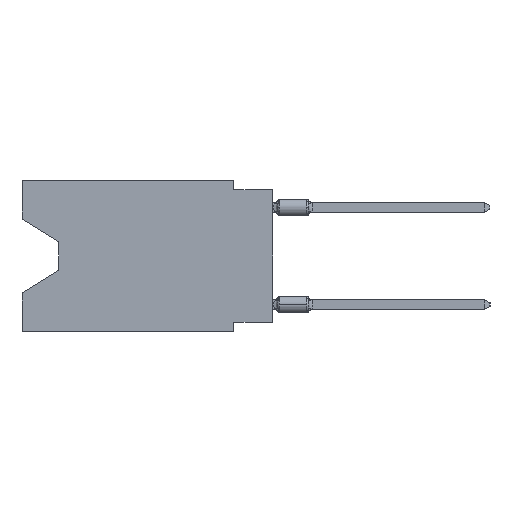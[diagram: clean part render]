
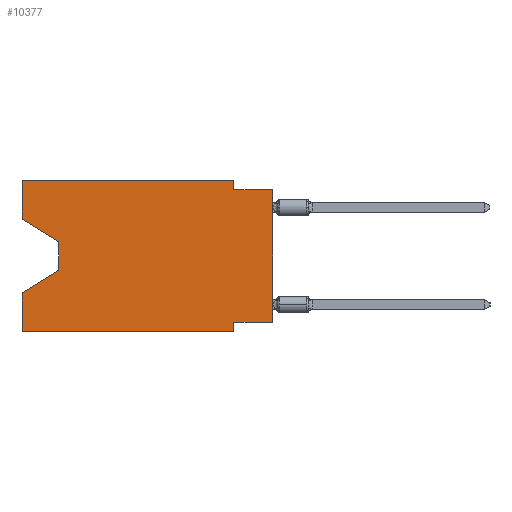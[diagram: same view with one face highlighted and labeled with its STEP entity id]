
A CAD part, left-side view. The second image highlights one B-rep face of the part: STEP entity #10377.
In plain terms, the highlighted planar face has unit normal (-1, 0, 0).
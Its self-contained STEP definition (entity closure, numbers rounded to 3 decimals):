
#88 = LINE ( 'NONE', #32011, #31797 ) ;
#122 = DIRECTION ( 'NONE',  ( 0., 0., 1. ) ) ;
#238 = LINE ( 'NONE', #20340, #31141 ) ;
#294 = DIRECTION ( 'NONE',  ( 0., 1., 0. ) ) ;
#889 = DIRECTION ( 'NONE',  ( 0., 0., -1. ) ) ;
#979 = DIRECTION ( 'NONE',  ( 0., 0.855, -0.519 ) ) ;
#1018 = VECTOR ( 'NONE', #294, 1000. ) ;
#1176 = CARTESIAN_POINT ( 'NONE',  ( 0., 16.383, 0. ) ) ;
#1333 = CARTESIAN_POINT ( 'NONE',  ( 0., 13.97, -4.013 ) ) ;
#1565 = EDGE_CURVE ( 'NONE', #36965, #25003, #2427, .T. ) ;
#2427 = LINE ( 'NONE', #22692, #28258 ) ;
#3397 = CARTESIAN_POINT ( 'NONE',  ( 0., 0., -9.271 ) ) ;
#3689 = CARTESIAN_POINT ( 'NONE',  ( 0., 2.54, -0.635 ) ) ;
#3773 = EDGE_CURVE ( 'NONE', #7853, #16053, #88, .T. ) ;
#4443 = DIRECTION ( 'NONE',  ( 0., 0., 1. ) ) ;
#4765 = VECTOR ( 'NONE', #889, 1000. ) ;
#4847 = VERTEX_POINT ( 'NONE', #28149 ) ;
#4906 = DIRECTION ( 'NONE',  ( 0., 0., -1. ) ) ;
#5166 = VECTOR ( 'NONE', #4443, 1000. ) ;
#5516 = ORIENTED_EDGE ( 'NONE', *, *, #20604, .T. ) ;
#5709 = LINE ( 'NONE', #32572, #13182 ) ;
#6017 = ORIENTED_EDGE ( 'NONE', *, *, #27268, .F. ) ;
#6082 = ORIENTED_EDGE ( 'NONE', *, *, #20113, .T. ) ;
#6728 = LINE ( 'NONE', #30863, #16703 ) ;
#7467 = LINE ( 'NONE', #34521, #18768 ) ;
#7670 = ORIENTED_EDGE ( 'NONE', *, *, #17733, .F. ) ;
#7853 = VERTEX_POINT ( 'NONE', #1333 ) ;
#8431 = DIRECTION ( 'NONE',  ( 0., 0., -1. ) ) ;
#9542 = CARTESIAN_POINT ( 'NONE',  ( 0., 0., -9.271 ) ) ;
#9868 = ORIENTED_EDGE ( 'NONE', *, *, #16961, .F. ) ;
#10208 = ORIENTED_EDGE ( 'NONE', *, *, #37325, .F. ) ;
#10320 = PLANE ( 'NONE',  #21846 ) ;
#10377 = ADVANCED_FACE ( 'NONE', ( #13979 ), #10320, .F. ) ;
#10885 = DIRECTION ( 'NONE',  ( 1., 0., 0. ) ) ;
#11122 = CARTESIAN_POINT ( 'NONE',  ( 0., 2.54, -9.271 ) ) ;
#11382 = ORIENTED_EDGE ( 'NONE', *, *, #1565, .F. ) ;
#12077 = DIRECTION ( 'NONE',  ( 0., -1., 0. ) ) ;
#12744 = LINE ( 'NONE', #33243, #15649 ) ;
#12853 = LINE ( 'NONE', #21547, #4765 ) ;
#12995 = VERTEX_POINT ( 'NONE', #36056 ) ;
#13182 = VECTOR ( 'NONE', #35274, 1000. ) ;
#13979 = FACE_OUTER_BOUND ( 'NONE', #22973, .T. ) ;
#15639 = ORIENTED_EDGE ( 'NONE', *, *, #19374, .T. ) ;
#15649 = VECTOR ( 'NONE', #979, 1000. ) ;
#16053 = VERTEX_POINT ( 'NONE', #17412 ) ;
#16703 = VECTOR ( 'NONE', #28278, 1000. ) ;
#16961 = EDGE_CURVE ( 'NONE', #12995, #26258, #25131, .T. ) ;
#17412 = CARTESIAN_POINT ( 'NONE',  ( 0., 13.97, -5.893 ) ) ;
#17643 = DIRECTION ( 'NONE',  ( 0., -0.855, -0.519 ) ) ;
#17688 = LINE ( 'NONE', #28387, #28089 ) ;
#17733 = EDGE_CURVE ( 'NONE', #34041, #21862, #26771, .T. ) ;
#18297 = LINE ( 'NONE', #29891, #20986 ) ;
#18768 = VECTOR ( 'NONE', #25828, 1000. ) ;
#19374 = EDGE_CURVE ( 'NONE', #16053, #26258, #12744, .T. ) ;
#19878 = EDGE_CURVE ( 'NONE', #25003, #28937, #7467, .T. ) ;
#20113 = EDGE_CURVE ( 'NONE', #34041, #28937, #5709, .T. ) ;
#20340 = CARTESIAN_POINT ( 'NONE',  ( 0., 16.383, -2.546 ) ) ;
#20567 = CARTESIAN_POINT ( 'NONE',  ( 0., 16.383, -2.546 ) ) ;
#20604 = EDGE_CURVE ( 'NONE', #24262, #7853, #238, .T. ) ;
#20986 = VECTOR ( 'NONE', #122, 1000. ) ;
#21547 = CARTESIAN_POINT ( 'NONE',  ( 0., 2.54, -9.906 ) ) ;
#21846 = AXIS2_PLACEMENT_3D ( 'NONE', #34278, #10885, #4906 ) ;
#21862 = VERTEX_POINT ( 'NONE', #11122 ) ;
#22692 = CARTESIAN_POINT ( 'NONE',  ( 0., 2.54, 0. ) ) ;
#22973 = EDGE_LOOP ( 'NONE', ( #5516, #37723, #15639, #9868, #28539, #6017, #7670, #6082, #28277, #11382, #23898, #10208 ) ) ;
#23240 = CARTESIAN_POINT ( 'NONE',  ( 0., 2.54, -9.906 ) ) ;
#23898 = ORIENTED_EDGE ( 'NONE', *, *, #25287, .F. ) ;
#24262 = VERTEX_POINT ( 'NONE', #20567 ) ;
#25003 = VERTEX_POINT ( 'NONE', #3689 ) ;
#25105 = CARTESIAN_POINT ( 'NONE',  ( 0., 2.54, 0. ) ) ;
#25131 = LINE ( 'NONE', #1176, #5166 ) ;
#25287 = EDGE_CURVE ( 'NONE', #4847, #36965, #17688, .T. ) ;
#25499 = CARTESIAN_POINT ( 'NONE',  ( 0., 16.383, -7.36 ) ) ;
#25828 = DIRECTION ( 'NONE',  ( 0., -1., 0. ) ) ;
#26258 = VERTEX_POINT ( 'NONE', #25499 ) ;
#26771 = LINE ( 'NONE', #3397, #1018 ) ;
#27164 = CARTESIAN_POINT ( 'NONE',  ( 0., 0., -0.635 ) ) ;
#27268 = EDGE_CURVE ( 'NONE', #21862, #36280, #12853, .T. ) ;
#28089 = VECTOR ( 'NONE', #12077, 1000. ) ;
#28149 = CARTESIAN_POINT ( 'NONE',  ( 0., 16.383, 0. ) ) ;
#28258 = VECTOR ( 'NONE', #28886, 1000. ) ;
#28277 = ORIENTED_EDGE ( 'NONE', *, *, #19878, .F. ) ;
#28278 = DIRECTION ( 'NONE',  ( 0., -1., 0. ) ) ;
#28387 = CARTESIAN_POINT ( 'NONE',  ( 0., 16.383, 0. ) ) ;
#28539 = ORIENTED_EDGE ( 'NONE', *, *, #36065, .T. ) ;
#28886 = DIRECTION ( 'NONE',  ( 0., 0., -1. ) ) ;
#28937 = VERTEX_POINT ( 'NONE', #27164 ) ;
#29891 = CARTESIAN_POINT ( 'NONE',  ( 0., 16.383, 0. ) ) ;
#30863 = CARTESIAN_POINT ( 'NONE',  ( 0., 16.383, -9.906 ) ) ;
#31141 = VECTOR ( 'NONE', #17643, 1000. ) ;
#31797 = VECTOR ( 'NONE', #8431, 1000. ) ;
#32011 = CARTESIAN_POINT ( 'NONE',  ( 0., 13.97, -4.013 ) ) ;
#32572 = CARTESIAN_POINT ( 'NONE',  ( 0., 0., 0. ) ) ;
#33243 = CARTESIAN_POINT ( 'NONE',  ( 0., 13.97, -5.893 ) ) ;
#34041 = VERTEX_POINT ( 'NONE', #9542 ) ;
#34278 = CARTESIAN_POINT ( 'NONE',  ( 0., 16.383, 0. ) ) ;
#34521 = CARTESIAN_POINT ( 'NONE',  ( 0., 0., -0.635 ) ) ;
#35274 = DIRECTION ( 'NONE',  ( 0., 0., 1. ) ) ;
#36056 = CARTESIAN_POINT ( 'NONE',  ( 0., 16.383, -9.906 ) ) ;
#36065 = EDGE_CURVE ( 'NONE', #12995, #36280, #6728, .T. ) ;
#36280 = VERTEX_POINT ( 'NONE', #23240 ) ;
#36965 = VERTEX_POINT ( 'NONE', #25105 ) ;
#37325 = EDGE_CURVE ( 'NONE', #24262, #4847, #18297, .T. ) ;
#37723 = ORIENTED_EDGE ( 'NONE', *, *, #3773, .T. ) ;
